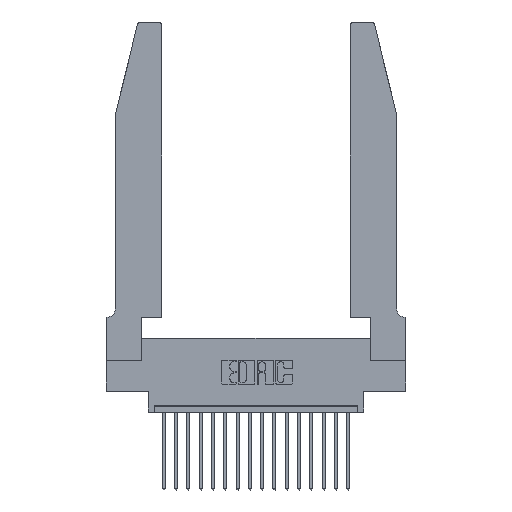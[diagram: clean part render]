
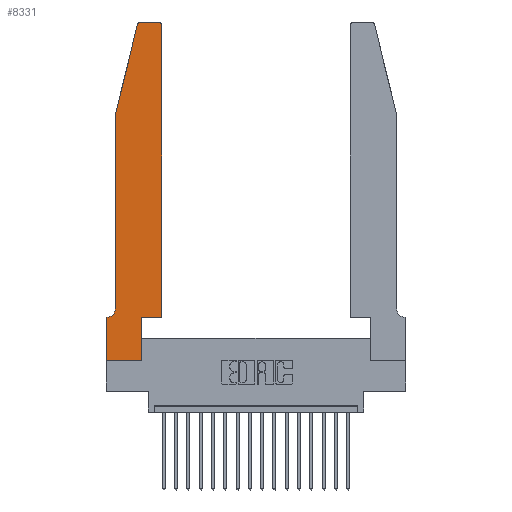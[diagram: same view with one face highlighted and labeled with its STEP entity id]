
A CAD part, top view. The second image highlights one B-rep face of the part: STEP entity #8331.
In plain terms, the highlighted planar face has unit normal (0, 0, 1).
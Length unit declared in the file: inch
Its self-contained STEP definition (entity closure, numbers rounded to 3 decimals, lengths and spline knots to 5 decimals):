
#8 = DIRECTION ( 'NONE',  ( -1., 0., 0. ) ) ;
#706 = VERTEX_POINT ( 'NONE', #19565 ) ;
#711 = DIRECTION ( 'NONE',  ( -1., 0., 0. ) ) ;
#2104 = CARTESIAN_POINT ( 'NONE',  ( 0.2605, 2.75, 0.37 ) ) ;
#2363 = VECTOR ( 'NONE', #17208, 39.37008 ) ;
#2644 = EDGE_CURVE ( 'NONE', #4536, #6245, #13454, .T. ) ;
#3082 = CARTESIAN_POINT ( 'NONE',  ( 0., 0., 0.37 ) ) ;
#3202 = CARTESIAN_POINT ( 'NONE',  ( 0., 0.35, 0.37 ) ) ;
#3419 = DIRECTION ( 'NONE',  ( 0., 0., 1. ) ) ;
#3524 = CARTESIAN_POINT ( 'NONE',  ( 0.2865, 0.35, 0.37 ) ) ;
#4031 = ORIENTED_EDGE ( 'NONE', *, *, #6365, .T. ) ;
#4282 = CARTESIAN_POINT ( 'NONE',  ( 0.0755, 0.35, 0.37 ) ) ;
#4535 = VERTEX_POINT ( 'NONE', #9799 ) ;
#4536 = VERTEX_POINT ( 'NONE', #6829 ) ;
#4582 = EDGE_CURVE ( 'NONE', #4535, #12016, #8506, .T. ) ;
#4786 = DIRECTION ( 'NONE',  ( 0., 0., 1. ) ) ;
#4868 = ORIENTED_EDGE ( 'NONE', *, *, #19917, .T. ) ;
#5001 = CARTESIAN_POINT ( 'NONE',  ( 0., 0.35, 0.37 ) ) ;
#5138 = DIRECTION ( 'NONE',  ( 1., 0., 0. ) ) ;
#5307 = DIRECTION ( 'NONE',  ( -1., 0., 0. ) ) ;
#5778 = DIRECTION ( 'NONE',  ( -0.239, -0.971, 0. ) ) ;
#5938 = DIRECTION ( 'NONE',  ( 0., -1., 0. ) ) ;
#6141 = LINE ( 'NONE', #13752, #15507 ) ;
#6182 = LINE ( 'NONE', #10265, #8419 ) ;
#6197 = VECTOR ( 'NONE', #11137, 39.37008 ) ;
#6245 = VERTEX_POINT ( 'NONE', #7507 ) ;
#6301 = VERTEX_POINT ( 'NONE', #7990 ) ;
#6308 = EDGE_CURVE ( 'NONE', #7672, #19625, #13096, .T. ) ;
#6319 = ORIENTED_EDGE ( 'NONE', *, *, #6648, .T. ) ;
#6365 = EDGE_CURVE ( 'NONE', #9575, #12256, #6182, .T. ) ;
#6648 = EDGE_CURVE ( 'NONE', #19123, #706, #19745, .T. ) ;
#6734 = CARTESIAN_POINT ( 'NONE',  ( 0.284, 2.72, 0.37 ) ) ;
#6829 = CARTESIAN_POINT ( 'NONE',  ( 0.4505, 0.35, 0.37 ) ) ;
#7051 = CARTESIAN_POINT ( 'NONE',  ( 0.0755, 2., 0.37 ) ) ;
#7068 = LINE ( 'NONE', #3082, #2363 ) ;
#7507 = CARTESIAN_POINT ( 'NONE',  ( 0.4505, 2.72, 0.37 ) ) ;
#7672 = VERTEX_POINT ( 'NONE', #8010 ) ;
#7680 = ORIENTED_EDGE ( 'NONE', *, *, #16012, .T. ) ;
#7896 = CARTESIAN_POINT ( 'NONE',  ( 0.0055, 0.42, 0.37 ) ) ;
#7990 = CARTESIAN_POINT ( 'NONE',  ( 0.4205, 2.75, 0.37 ) ) ;
#8010 = CARTESIAN_POINT ( 'NONE',  ( 0.284, 2.75, 0.37 ) ) ;
#8266 = VECTOR ( 'NONE', #9941, 39.37008 ) ;
#8331 = ADVANCED_FACE ( 'NONE', ( #9584 ), #17555, .T. ) ;
#8334 = DIRECTION ( 'NONE',  ( 0., 0., 1. ) ) ;
#8411 = EDGE_CURVE ( 'NONE', #6301, #7672, #12284, .T. ) ;
#8419 = VECTOR ( 'NONE', #15072, 39.37008 ) ;
#8506 = LINE ( 'NONE', #4282, #11723 ) ;
#8810 = EDGE_CURVE ( 'NONE', #706, #4535, #12026, .T. ) ;
#9047 = CARTESIAN_POINT ( 'NONE',  ( 0.0755, 2., 0.37 ) ) ;
#9575 = VERTEX_POINT ( 'NONE', #18485 ) ;
#9584 = FACE_OUTER_BOUND ( 'NONE', #17581, .T. ) ;
#9799 = CARTESIAN_POINT ( 'NONE',  ( 0.0055, 0.35, 0.37 ) ) ;
#9941 = DIRECTION ( 'NONE',  ( 0., 1., 0. ) ) ;
#10146 = LINE ( 'NONE', #17186, #6197 ) ;
#10265 = CARTESIAN_POINT ( 'NONE',  ( 0., 0., 0.37 ) ) ;
#10529 = DIRECTION ( 'NONE',  ( 0., 1., 0. ) ) ;
#10622 = ORIENTED_EDGE ( 'NONE', *, *, #2644, .T. ) ;
#11037 = ORIENTED_EDGE ( 'NONE', *, *, #8411, .T. ) ;
#11137 = DIRECTION ( 'NONE',  ( 1., 0., 0. ) ) ;
#11146 = AXIS2_PLACEMENT_3D ( 'NONE', #6734, #8334, #16225 ) ;
#11723 = VECTOR ( 'NONE', #5307, 39.37008 ) ;
#12002 = EDGE_CURVE ( 'NONE', #6245, #6301, #20248, .T. ) ;
#12016 = VERTEX_POINT ( 'NONE', #3202 ) ;
#12026 = CIRCLE ( 'NONE', #19129, 0.07 ) ;
#12256 = VERTEX_POINT ( 'NONE', #17631 ) ;
#12284 = LINE ( 'NONE', #2104, #15970 ) ;
#13007 = ORIENTED_EDGE ( 'NONE', *, *, #18936, .T. ) ;
#13096 = CIRCLE ( 'NONE', #11146, 0.03 ) ;
#13413 = LINE ( 'NONE', #3524, #8266 ) ;
#13454 = LINE ( 'NONE', #18180, #17165 ) ;
#13752 = CARTESIAN_POINT ( 'NONE',  ( 0.0755, 2., 0.37 ) ) ;
#14381 = ORIENTED_EDGE ( 'NONE', *, *, #6308, .T. ) ;
#14413 = DIRECTION ( 'NONE',  ( 0., 0., -1. ) ) ;
#15072 = DIRECTION ( 'NONE',  ( 1., 0., 0. ) ) ;
#15161 = EDGE_CURVE ( 'NONE', #12016, #9575, #7068, .T. ) ;
#15211 = VERTEX_POINT ( 'NONE', #18797 ) ;
#15357 = CARTESIAN_POINT ( 'NONE',  ( 0.4205, 2.72, 0.37 ) ) ;
#15376 = ORIENTED_EDGE ( 'NONE', *, *, #4582, .T. ) ;
#15507 = VECTOR ( 'NONE', #5778, 39.37008 ) ;
#15970 = VECTOR ( 'NONE', #711, 39.37008 ) ;
#16012 = EDGE_CURVE ( 'NONE', #12256, #15211, #13413, .T. ) ;
#16225 = DIRECTION ( 'NONE',  ( 1., 0., 0. ) ) ;
#16625 = ORIENTED_EDGE ( 'NONE', *, *, #8810, .T. ) ;
#17165 = VECTOR ( 'NONE', #10529, 39.37008 ) ;
#17186 = CARTESIAN_POINT ( 'NONE',  ( 0.4505, 0.35, 0.37 ) ) ;
#17208 = DIRECTION ( 'NONE',  ( 0., -1., 0. ) ) ;
#17218 = ORIENTED_EDGE ( 'NONE', *, *, #12002, .T. ) ;
#17366 = CARTESIAN_POINT ( 'NONE',  ( 0.25487, 2.72718, 0.37 ) ) ;
#17408 = AXIS2_PLACEMENT_3D ( 'NONE', #5001, #3419, #5138 ) ;
#17538 = DIRECTION ( 'NONE',  ( 1., 0., 0. ) ) ;
#17555 = PLANE ( 'NONE',  #17408 ) ;
#17581 = EDGE_LOOP ( 'NONE', ( #11037, #14381, #4868, #6319, #16625, #15376, #18173, #4031, #7680, #13007, #10622, #17218 ) ) ;
#17631 = CARTESIAN_POINT ( 'NONE',  ( 0.2865, 0., 0.37 ) ) ;
#18173 = ORIENTED_EDGE ( 'NONE', *, *, #15161, .T. ) ;
#18180 = CARTESIAN_POINT ( 'NONE',  ( 0.4505, 0.35, 0.37 ) ) ;
#18485 = CARTESIAN_POINT ( 'NONE',  ( 0., 0., 0.37 ) ) ;
#18797 = CARTESIAN_POINT ( 'NONE',  ( 0.2865, 0.35, 0.37 ) ) ;
#18936 = EDGE_CURVE ( 'NONE', #15211, #4536, #10146, .T. ) ;
#19005 = VECTOR ( 'NONE', #5938, 39.37008 ) ;
#19123 = VERTEX_POINT ( 'NONE', #7051 ) ;
#19129 = AXIS2_PLACEMENT_3D ( 'NONE', #7896, #14413, #8 ) ;
#19565 = CARTESIAN_POINT ( 'NONE',  ( 0.0755, 0.42, 0.37 ) ) ;
#19625 = VERTEX_POINT ( 'NONE', #17366 ) ;
#19745 = LINE ( 'NONE', #9047, #19005 ) ;
#19866 = AXIS2_PLACEMENT_3D ( 'NONE', #15357, #4786, #17538 ) ;
#19917 = EDGE_CURVE ( 'NONE', #19625, #19123, #6141, .T. ) ;
#20248 = CIRCLE ( 'NONE', #19866, 0.03 ) ;
